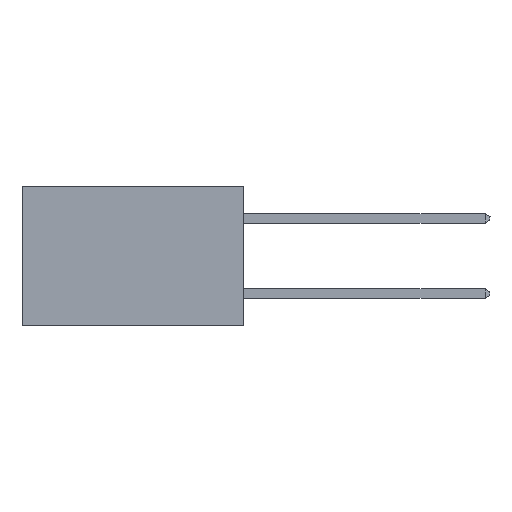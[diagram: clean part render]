
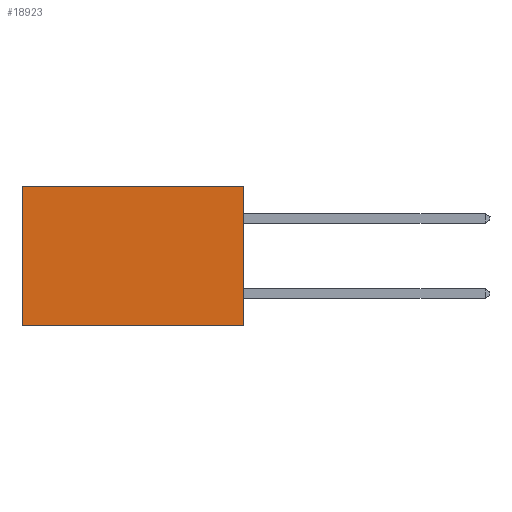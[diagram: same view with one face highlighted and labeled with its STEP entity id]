
A CAD part, left-side view. The second image highlights one B-rep face of the part: STEP entity #18923.
In plain terms, the highlighted planar face has unit normal (-1, 0, 0).
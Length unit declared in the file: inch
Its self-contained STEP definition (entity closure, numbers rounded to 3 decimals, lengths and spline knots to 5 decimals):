
#192 = ORIENTED_EDGE ( 'NONE', *, *, #4786, .T. ) ;
#612 = ORIENTED_EDGE ( 'NONE', *, *, #14693, .F. ) ;
#1207 = CARTESIAN_POINT ( 'NONE',  ( 0.277, 0., -0.37 ) ) ;
#1323 = EDGE_LOOP ( 'NONE', ( #3018, #612, #4843, #192 ) ) ;
#1900 = VERTEX_POINT ( 'NONE', #13622 ) ;
#2390 = EDGE_CURVE ( 'NONE', #1900, #16732, #5817, .T. ) ;
#3018 = ORIENTED_EDGE ( 'NONE', *, *, #2390, .T. ) ;
#3236 = FACE_OUTER_BOUND ( 'NONE', #1323, .T. ) ;
#3743 = AXIS2_PLACEMENT_3D ( 'NONE', #13507, #4323, #15070 ) ;
#3931 = LINE ( 'NONE', #12807, #12121 ) ;
#4126 = LINE ( 'NONE', #1207, #6169 ) ;
#4323 = DIRECTION ( 'NONE',  ( 1., 0., 0. ) ) ;
#4399 = CARTESIAN_POINT ( 'NONE',  ( 0.277, 0.59, -0.37 ) ) ;
#4786 = EDGE_CURVE ( 'NONE', #18064, #1900, #3931, .T. ) ;
#4843 = ORIENTED_EDGE ( 'NONE', *, *, #6719, .F. ) ;
#5345 = VECTOR ( 'NONE', #7365, 39.37008 ) ;
#5372 = VECTOR ( 'NONE', #18508, 39.37008 ) ;
#5817 = LINE ( 'NONE', #7190, #5345 ) ;
#5996 = CARTESIAN_POINT ( 'NONE',  ( 0.277, 0., -0.37 ) ) ;
#6169 = VECTOR ( 'NONE', #11986, 39.37008 ) ;
#6719 = EDGE_CURVE ( 'NONE', #18064, #7148, #4126, .T. ) ;
#7148 = VERTEX_POINT ( 'NONE', #12976 ) ;
#7190 = CARTESIAN_POINT ( 'NONE',  ( 0.277, 0.59, -0.37 ) ) ;
#7365 = DIRECTION ( 'NONE',  ( 0., 0., -1. ) ) ;
#8780 = CARTESIAN_POINT ( 'NONE',  ( 0.277, 0., 0. ) ) ;
#10390 = PLANE ( 'NONE',  #3743 ) ;
#11986 = DIRECTION ( 'NONE',  ( 0., 0., -1. ) ) ;
#12121 = VECTOR ( 'NONE', #12793, 39.37008 ) ;
#12793 = DIRECTION ( 'NONE',  ( 0., 1., 0. ) ) ;
#12807 = CARTESIAN_POINT ( 'NONE',  ( 0.277, 0., 0. ) ) ;
#12976 = CARTESIAN_POINT ( 'NONE',  ( 0.277, 0., -0.37 ) ) ;
#13507 = CARTESIAN_POINT ( 'NONE',  ( 0.277, 0., -0.37 ) ) ;
#13622 = CARTESIAN_POINT ( 'NONE',  ( 0.277, 0.59, 0. ) ) ;
#14693 = EDGE_CURVE ( 'NONE', #7148, #16732, #17686, .T. ) ;
#15070 = DIRECTION ( 'NONE',  ( 0., 0., -1. ) ) ;
#16732 = VERTEX_POINT ( 'NONE', #4399 ) ;
#17686 = LINE ( 'NONE', #5996, #5372 ) ;
#18064 = VERTEX_POINT ( 'NONE', #8780 ) ;
#18508 = DIRECTION ( 'NONE',  ( 0., 1., 0. ) ) ;
#18923 = ADVANCED_FACE ( 'NONE', ( #3236 ), #10390, .F. ) ;
